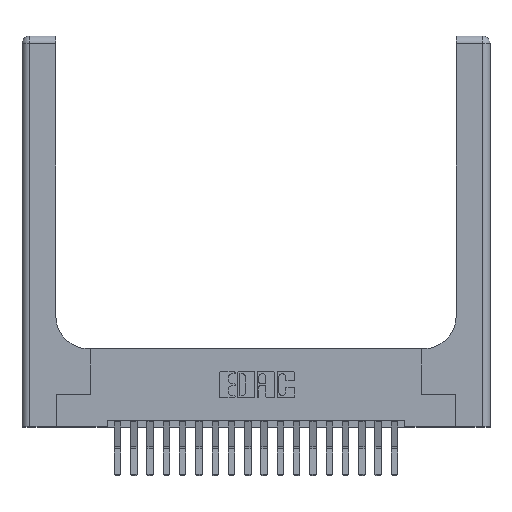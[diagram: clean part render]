
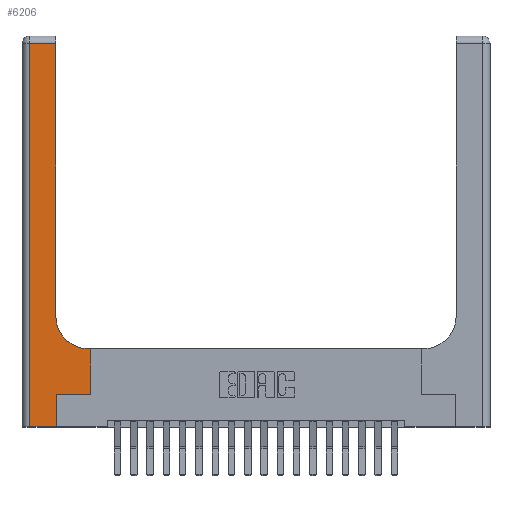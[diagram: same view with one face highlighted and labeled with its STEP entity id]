
A CAD part, top view. The second image highlights one B-rep face of the part: STEP entity #6206.
In plain terms, the highlighted planar face has unit normal (0, 0, 1).
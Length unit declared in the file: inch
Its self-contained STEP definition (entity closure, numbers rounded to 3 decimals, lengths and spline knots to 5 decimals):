
#299 = DIRECTION ( 'NONE',  ( 1., 0., 0. ) ) ;
#397 = ORIENTED_EDGE ( 'NONE', *, *, #16064, .T. ) ;
#1426 = CARTESIAN_POINT ( 'NONE',  ( 0.265, 0.25, 0.37 ) ) ;
#1701 = VECTOR ( 'NONE', #13732, 39.37008 ) ;
#1773 = CARTESIAN_POINT ( 'NONE',  ( 0.26, 0.85, 0.37 ) ) ;
#1833 = LINE ( 'NONE', #1426, #19441 ) ;
#2053 = EDGE_CURVE ( 'NONE', #16600, #7567, #14490, .T. ) ;
#2117 = LINE ( 'NONE', #8500, #6964 ) ;
#2558 = LINE ( 'NONE', #15291, #8507 ) ;
#2962 = CARTESIAN_POINT ( 'NONE',  ( 0.528, 0.25, 0.37 ) ) ;
#2964 = CARTESIAN_POINT ( 'NONE',  ( 0.265, 0., 0.37 ) ) ;
#3058 = VERTEX_POINT ( 'NONE', #9059 ) ;
#3145 = CARTESIAN_POINT ( 'NONE',  ( 0.06, 2.94, 0.37 ) ) ;
#3255 = EDGE_CURVE ( 'NONE', #7567, #9006, #20133, .T. ) ;
#4096 = CARTESIAN_POINT ( 'NONE',  ( 0., 3., 0.37 ) ) ;
#4415 = DIRECTION ( 'NONE',  ( 0., 0., -1. ) ) ;
#4421 = EDGE_CURVE ( 'NONE', #12890, #20243, #1833, .T. ) ;
#4752 = VECTOR ( 'NONE', #7070, 39.37008 ) ;
#5031 = ORIENTED_EDGE ( 'NONE', *, *, #13503, .T. ) ;
#5033 = FACE_OUTER_BOUND ( 'NONE', #9903, .T. ) ;
#5426 = CARTESIAN_POINT ( 'NONE',  ( 0.51, 0.85, 0.37 ) ) ;
#5505 = LINE ( 'NONE', #16668, #1701 ) ;
#6074 = EDGE_CURVE ( 'NONE', #3058, #12890, #17551, .T. ) ;
#6206 = ADVANCED_FACE ( 'NONE', ( #5033 ), #11610, .F. ) ;
#6964 = VECTOR ( 'NONE', #13309, 39.37008 ) ;
#7039 = CARTESIAN_POINT ( 'NONE',  ( 0.26, 2.94, 0.37 ) ) ;
#7070 = DIRECTION ( 'NONE',  ( 0., -1., 0. ) ) ;
#7160 = VECTOR ( 'NONE', #14316, 39.37008 ) ;
#7525 = ORIENTED_EDGE ( 'NONE', *, *, #4421, .T. ) ;
#7567 = VERTEX_POINT ( 'NONE', #3145 ) ;
#7707 = ORIENTED_EDGE ( 'NONE', *, *, #18782, .T. ) ;
#7817 = DIRECTION ( 'NONE',  ( 1., 0., 0. ) ) ;
#7820 = ORIENTED_EDGE ( 'NONE', *, *, #6074, .T. ) ;
#8288 = VERTEX_POINT ( 'NONE', #14170 ) ;
#8494 = ORIENTED_EDGE ( 'NONE', *, *, #8798, .T. ) ;
#8500 = CARTESIAN_POINT ( 'NONE',  ( 0.26, 0.6, 0.37 ) ) ;
#8507 = VECTOR ( 'NONE', #299, 39.37008 ) ;
#8700 = AXIS2_PLACEMENT_3D ( 'NONE', #5426, #8772, #16702 ) ;
#8705 = VECTOR ( 'NONE', #9427, 39.37008 ) ;
#8772 = DIRECTION ( 'NONE',  ( 0., 0., -1. ) ) ;
#8798 = EDGE_CURVE ( 'NONE', #9006, #3058, #2558, .T. ) ;
#8878 = ORIENTED_EDGE ( 'NONE', *, *, #3255, .T. ) ;
#9006 = VERTEX_POINT ( 'NONE', #18245 ) ;
#9059 = CARTESIAN_POINT ( 'NONE',  ( 0.265, 0., 0.37 ) ) ;
#9427 = DIRECTION ( 'NONE',  ( -1., 0., 0. ) ) ;
#9903 = EDGE_LOOP ( 'NONE', ( #397, #11805, #8878, #8494, #7820, #7525, #11099, #5031, #7707 ) ) ;
#10010 = LINE ( 'NONE', #11678, #12692 ) ;
#10723 = CIRCLE ( 'NONE', #8700, 0.25 ) ;
#11099 = ORIENTED_EDGE ( 'NONE', *, *, #18994, .T. ) ;
#11381 = DIRECTION ( 'NONE',  ( 0., 1., 0. ) ) ;
#11610 = PLANE ( 'NONE',  #16454 ) ;
#11678 = CARTESIAN_POINT ( 'NONE',  ( 0.26, 3., 0.37 ) ) ;
#11805 = ORIENTED_EDGE ( 'NONE', *, *, #2053, .T. ) ;
#11810 = VERTEX_POINT ( 'NONE', #1773 ) ;
#12692 = VECTOR ( 'NONE', #11381, 39.37008 ) ;
#12886 = CARTESIAN_POINT ( 'NONE',  ( 0.265, 0.25, 0.37 ) ) ;
#12890 = VERTEX_POINT ( 'NONE', #12886 ) ;
#13309 = DIRECTION ( 'NONE',  ( -1., 0., 0. ) ) ;
#13503 = EDGE_CURVE ( 'NONE', #8288, #15780, #2117, .T. ) ;
#13732 = DIRECTION ( 'NONE',  ( 0., 1., 0. ) ) ;
#14170 = CARTESIAN_POINT ( 'NONE',  ( 0.528, 0.6, 0.37 ) ) ;
#14316 = DIRECTION ( 'NONE',  ( 0., 1., 0. ) ) ;
#14490 = LINE ( 'NONE', #19197, #8705 ) ;
#15291 = CARTESIAN_POINT ( 'NONE',  ( 0., 0., 0.37 ) ) ;
#15780 = VERTEX_POINT ( 'NONE', #17870 ) ;
#16064 = EDGE_CURVE ( 'NONE', #11810, #16600, #10010, .T. ) ;
#16454 = AXIS2_PLACEMENT_3D ( 'NONE', #4096, #4415, #20279 ) ;
#16600 = VERTEX_POINT ( 'NONE', #7039 ) ;
#16668 = CARTESIAN_POINT ( 'NONE',  ( 0.528, 0.25, 0.37 ) ) ;
#16702 = DIRECTION ( 'NONE',  ( 1., 0., 0. ) ) ;
#17551 = LINE ( 'NONE', #2964, #7160 ) ;
#17870 = CARTESIAN_POINT ( 'NONE',  ( 0.51, 0.6, 0.37 ) ) ;
#18245 = CARTESIAN_POINT ( 'NONE',  ( 0.06, 0., 0.37 ) ) ;
#18782 = EDGE_CURVE ( 'NONE', #15780, #11810, #10723, .T. ) ;
#18994 = EDGE_CURVE ( 'NONE', #20243, #8288, #5505, .T. ) ;
#19197 = CARTESIAN_POINT ( 'NONE',  ( 0., 2.94, 0.37 ) ) ;
#19441 = VECTOR ( 'NONE', #7817, 39.37008 ) ;
#20133 = LINE ( 'NONE', #20240, #4752 ) ;
#20240 = CARTESIAN_POINT ( 'NONE',  ( 0.06, 3., 0.37 ) ) ;
#20243 = VERTEX_POINT ( 'NONE', #2962 ) ;
#20279 = DIRECTION ( 'NONE',  ( -1., 0., 0. ) ) ;
